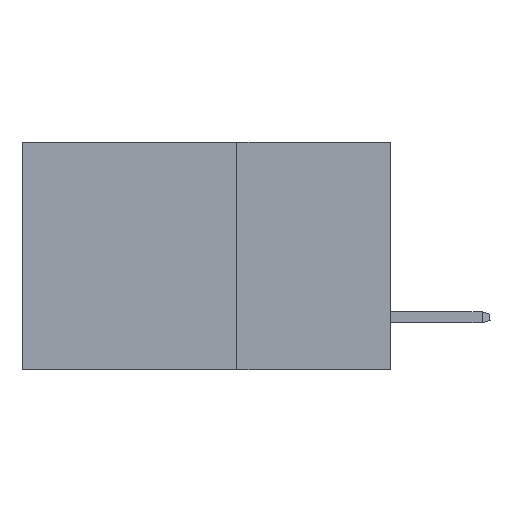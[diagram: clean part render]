
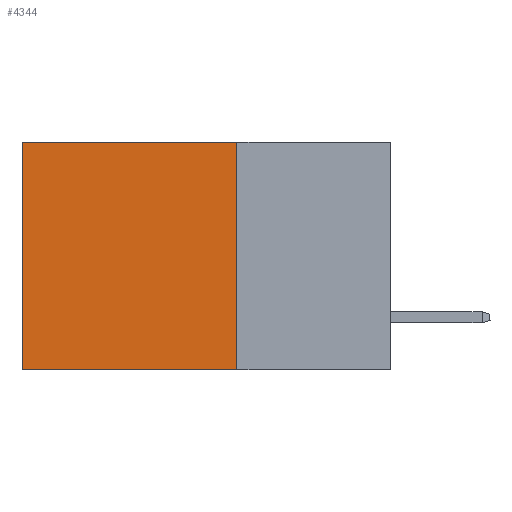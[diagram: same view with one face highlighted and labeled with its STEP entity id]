
A CAD part, left-side view. The second image highlights one B-rep face of the part: STEP entity #4344.
In plain terms, the highlighted planar face has unit normal (-1, 0, 0).
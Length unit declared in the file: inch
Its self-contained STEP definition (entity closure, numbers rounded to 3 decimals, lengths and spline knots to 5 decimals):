
#35 = DIRECTION ( 'NONE',  ( 1., 0., 0. ) ) ;
#222 = CARTESIAN_POINT ( 'NONE',  ( 0.2875, 0.6, 0. ) ) ;
#555 = EDGE_CURVE ( 'NONE', #10293, #3792, #16849, .T. ) ;
#1264 = EDGE_CURVE ( 'NONE', #3368, #6389, #5197, .T. ) ;
#2641 = CARTESIAN_POINT ( 'NONE',  ( 0.2875, 0.6, -0.37 ) ) ;
#2699 = PLANE ( 'NONE',  #10103 ) ;
#3368 = VERTEX_POINT ( 'NONE', #222 ) ;
#3792 = VERTEX_POINT ( 'NONE', #12382 ) ;
#3831 = CARTESIAN_POINT ( 'NONE',  ( 0.2875, 0.25, -0.37 ) ) ;
#4344 = ADVANCED_FACE ( 'NONE', ( #13944 ), #2699, .F. ) ;
#4603 = LINE ( 'NONE', #3831, #5434 ) ;
#5120 = ORIENTED_EDGE ( 'NONE', *, *, #555, .F. ) ;
#5197 = LINE ( 'NONE', #14035, #8558 ) ;
#5335 = VECTOR ( 'NONE', #6800, 39.37008 ) ;
#5434 = VECTOR ( 'NONE', #6524, 39.37008 ) ;
#6389 = VERTEX_POINT ( 'NONE', #2641 ) ;
#6524 = DIRECTION ( 'NONE',  ( 0., 1., 0. ) ) ;
#6800 = DIRECTION ( 'NONE',  ( 0., 1., 0. ) ) ;
#7120 = ORIENTED_EDGE ( 'NONE', *, *, #15493, .T. ) ;
#7695 = EDGE_LOOP ( 'NONE', ( #13096, #10776, #5120, #7120 ) ) ;
#8038 = CARTESIAN_POINT ( 'NONE',  ( 0.2875, 0.25, 0. ) ) ;
#8558 = VECTOR ( 'NONE', #16859, 39.37008 ) ;
#9046 = CARTESIAN_POINT ( 'NONE',  ( 0.2875, 0.25, 0. ) ) ;
#9451 = EDGE_CURVE ( 'NONE', #3792, #6389, #4603, .T. ) ;
#10103 = AXIS2_PLACEMENT_3D ( 'NONE', #8038, #35, #16306 ) ;
#10135 = DIRECTION ( 'NONE',  ( 0., 0., -1. ) ) ;
#10293 = VERTEX_POINT ( 'NONE', #15128 ) ;
#10776 = ORIENTED_EDGE ( 'NONE', *, *, #9451, .F. ) ;
#12382 = CARTESIAN_POINT ( 'NONE',  ( 0.2875, 0.25, -0.37 ) ) ;
#13096 = ORIENTED_EDGE ( 'NONE', *, *, #1264, .T. ) ;
#13944 = FACE_OUTER_BOUND ( 'NONE', #7695, .T. ) ;
#14035 = CARTESIAN_POINT ( 'NONE',  ( 0.2875, 0.6, 0. ) ) ;
#14135 = CARTESIAN_POINT ( 'NONE',  ( 0.2875, 0.25, 0. ) ) ;
#15128 = CARTESIAN_POINT ( 'NONE',  ( 0.2875, 0.25, 0. ) ) ;
#15493 = EDGE_CURVE ( 'NONE', #10293, #3368, #15684, .T. ) ;
#15576 = VECTOR ( 'NONE', #10135, 39.37008 ) ;
#15684 = LINE ( 'NONE', #9046, #5335 ) ;
#16306 = DIRECTION ( 'NONE',  ( 0., 0., -1. ) ) ;
#16849 = LINE ( 'NONE', #14135, #15576 ) ;
#16859 = DIRECTION ( 'NONE',  ( 0., 0., -1. ) ) ;
